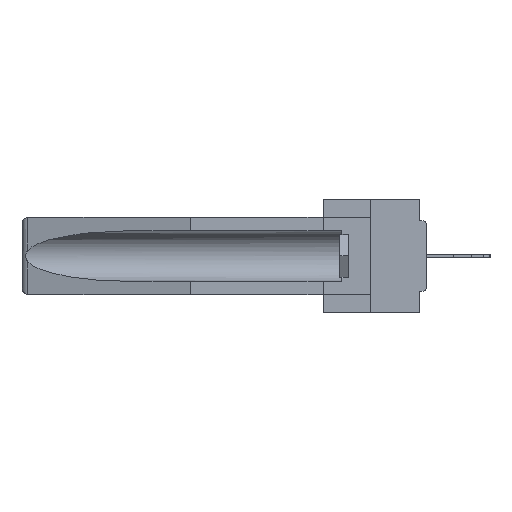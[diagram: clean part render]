
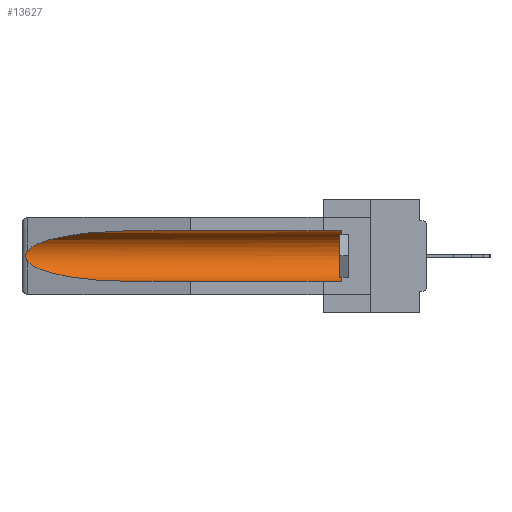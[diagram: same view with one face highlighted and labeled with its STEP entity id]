
A CAD part, left-side view. The second image highlights one B-rep face of the part: STEP entity #13627.
In plain terms, the highlighted cylindrical face has radius 2.857 mm (diameter 5.715 mm), a partial arc.
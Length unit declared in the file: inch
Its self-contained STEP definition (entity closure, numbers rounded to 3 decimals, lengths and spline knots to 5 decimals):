
#168 = AXIS2_PLACEMENT_3D ( 'NONE', #15860, #18467, #28395 ) ;
#196 = EDGE_CURVE ( 'NONE', #20129, #7748, #23588, .T. ) ;
#570 = B_SPLINE_CURVE_WITH_KNOTS ( 'NONE', 3,
 ( #27912, #25789, #28242, #11139, #20587, #1074, #10966, #15531, #28402, #12920 ),
 .UNSPECIFIED., .F., .F.,
 ( 4, 2, 2, 2, 4 ),
 ( 0., 0.00029, 0.00058, 0.00087, 0.00117 ),
 .UNSPECIFIED. ) ;
#593 = ORIENTED_EDGE ( 'NONE', *, *, #4536, .T. ) ;
#1074 = CARTESIAN_POINT ( 'NONE',  ( 0.2675, 1.53308, -0.17534 ) ) ;
#2402 = CARTESIAN_POINT ( 'NONE',  ( 0.155, 0.126, -0.059 ) ) ;
#2913 = CARTESIAN_POINT ( 'NONE',  ( 0.155, 0.126, -0.284 ) ) ;
#3176 = CARTESIAN_POINT ( 'NONE',  ( 0.21114, 1.30732, -0.284 ) ) ;
#4002 = ORIENTED_EDGE ( 'NONE', *, *, #28989, .T. ) ;
#4512 = EDGE_CURVE ( 'NONE', #31312, #16522, #10259, .T. ) ;
#4536 = EDGE_CURVE ( 'NONE', #16522, #20129, #570, .T. ) ;
#6184 = ORIENTED_EDGE ( 'NONE', *, *, #19245, .F. ) ;
#7378 = ORIENTED_EDGE ( 'NONE', *, *, #196, .T. ) ;
#7748 = VERTEX_POINT ( 'NONE', #11657 ) ;
#8348 = DIRECTION ( 'NONE',  ( 0., 1., 0. ) ) ;
#8386 = CARTESIAN_POINT ( 'NONE',  ( 0.25451, 1.48313, -0.09465 ) ) ;
#8705 = CARTESIAN_POINT ( 'NONE',  ( 0.21114, 1.30732, -0.059 ) ) ;
#8946 = CARTESIAN_POINT ( 'NONE',  ( 0.26537, 1.52718, -0.19328 ) ) ;
#8997 = VECTOR ( 'NONE', #28662, 39.37008 ) ;
#9002 = CYLINDRICAL_SURFACE ( 'NONE', #15094, 0.1125 ) ;
#10259 =( BOUNDED_CURVE ( )  B_SPLINE_CURVE ( 3, ( #16008, #8705, #8386, #25637 ),
 .UNSPECIFIED., .F., .T. ) 
 B_SPLINE_CURVE_WITH_KNOTS ( ( 4, 4 ),
 ( 4.71239, 6.08839 ),
 .UNSPECIFIED. ) 
 CURVE ( )  GEOMETRIC_REPRESENTATION_ITEM ( )  RATIONAL_B_SPLINE_CURVE ( ( 1., 0.848, 0.848, 1. ) ) 
 REPRESENTATION_ITEM ( '' )  );
#10966 = CARTESIAN_POINT ( 'NONE',  ( 0.2673, 1.53269, -0.17917 ) ) ;
#11139 = CARTESIAN_POINT ( 'NONE',  ( 0.2673, 1.5327, -0.16383 ) ) ;
#11610 = CARTESIAN_POINT ( 'NONE',  ( 0.155, -0.30754, -0.284 ) ) ;
#11657 = CARTESIAN_POINT ( 'NONE',  ( 0.155, 1.07973, -0.284 ) ) ;
#11773 = VERTEX_POINT ( 'NONE', #2913 ) ;
#12728 = LINE ( 'NONE', #16112, #8997 ) ;
#12920 = CARTESIAN_POINT ( 'NONE',  ( 0.26537, 1.52718, -0.19328 ) ) ;
#13219 = CARTESIAN_POINT ( 'NONE',  ( 0.155, -0.30754, -0.1715 ) ) ;
#13554 = VERTEX_POINT ( 'NONE', #2402 ) ;
#13627 = ADVANCED_FACE ( 'NONE', ( #18749 ), #9002, .F. ) ;
#15094 = AXIS2_PLACEMENT_3D ( 'NONE', #13219, #8348, #28204 ) ;
#15531 = CARTESIAN_POINT ( 'NONE',  ( 0.26655, 1.53094, -0.18657 ) ) ;
#15860 = CARTESIAN_POINT ( 'NONE',  ( 0.155, 0.126, -0.1715 ) ) ;
#16008 = CARTESIAN_POINT ( 'NONE',  ( 0.155, 1.07973, -0.059 ) ) ;
#16112 = CARTESIAN_POINT ( 'NONE',  ( 0.155, -0.30754, -0.059 ) ) ;
#16522 = VERTEX_POINT ( 'NONE', #18450 ) ;
#16809 = LINE ( 'NONE', #11610, #29836 ) ;
#17969 = CARTESIAN_POINT ( 'NONE',  ( 0.26537, 1.52718, -0.19328 ) ) ;
#18277 = EDGE_CURVE ( 'NONE', #13554, #31312, #12728, .T. ) ;
#18450 = CARTESIAN_POINT ( 'NONE',  ( 0.26537, 1.52718, -0.14972 ) ) ;
#18467 = DIRECTION ( 'NONE',  ( 0., -1., 0. ) ) ;
#18749 = FACE_OUTER_BOUND ( 'NONE', #18963, .T. ) ;
#18963 = EDGE_LOOP ( 'NONE', ( #27122, #593, #7378, #6184, #4002, #28065 ) ) ;
#19245 = EDGE_CURVE ( 'NONE', #11773, #7748, #16809, .T. ) ;
#20092 = CARTESIAN_POINT ( 'NONE',  ( 0.155, 1.07973, -0.284 ) ) ;
#20129 = VERTEX_POINT ( 'NONE', #8946 ) ;
#20587 = CARTESIAN_POINT ( 'NONE',  ( 0.2675, 1.53308, -0.16763 ) ) ;
#22703 = CARTESIAN_POINT ( 'NONE',  ( 0.25451, 1.48313, -0.24835 ) ) ;
#23588 =( BOUNDED_CURVE ( )  B_SPLINE_CURVE ( 3, ( #17969, #22703, #3176, #20092 ),
 .UNSPECIFIED., .F., .T. ) 
 B_SPLINE_CURVE_WITH_KNOTS ( ( 4, 4 ),
 ( 0.1948, 1.5708 ),
 .UNSPECIFIED. ) 
 CURVE ( )  GEOMETRIC_REPRESENTATION_ITEM ( )  RATIONAL_B_SPLINE_CURVE ( ( 1., 0.848, 0.848, 1. ) ) 
 REPRESENTATION_ITEM ( '' )  );
#24157 = DIRECTION ( 'NONE',  ( 0., 1., 0. ) ) ;
#25637 = CARTESIAN_POINT ( 'NONE',  ( 0.26537, 1.52718, -0.14972 ) ) ;
#25789 = CARTESIAN_POINT ( 'NONE',  ( 0.26597, 1.52961, -0.15275 ) ) ;
#25983 = CARTESIAN_POINT ( 'NONE',  ( 0.155, 1.07973, -0.059 ) ) ;
#27122 = ORIENTED_EDGE ( 'NONE', *, *, #4512, .T. ) ;
#27912 = CARTESIAN_POINT ( 'NONE',  ( 0.26537, 1.52718, -0.14972 ) ) ;
#28065 = ORIENTED_EDGE ( 'NONE', *, *, #18277, .T. ) ;
#28204 = DIRECTION ( 'NONE',  ( 0., 0., 1. ) ) ;
#28242 = CARTESIAN_POINT ( 'NONE',  ( 0.26654, 1.53092, -0.15636 ) ) ;
#28395 = DIRECTION ( 'NONE',  ( 0., 0., 1. ) ) ;
#28402 = CARTESIAN_POINT ( 'NONE',  ( 0.26597, 1.5296, -0.19026 ) ) ;
#28662 = DIRECTION ( 'NONE',  ( 0., 1., 0. ) ) ;
#28989 = EDGE_CURVE ( 'NONE', #11773, #13554, #30303, .T. ) ;
#29836 = VECTOR ( 'NONE', #24157, 39.37008 ) ;
#30303 = CIRCLE ( 'NONE', #168, 0.1125 ) ;
#31312 = VERTEX_POINT ( 'NONE', #25983 ) ;
